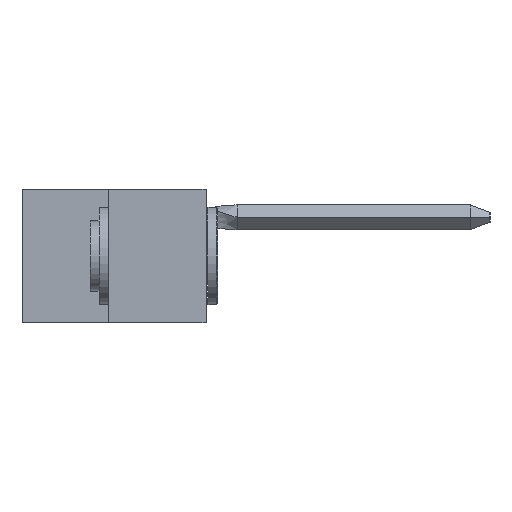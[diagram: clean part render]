
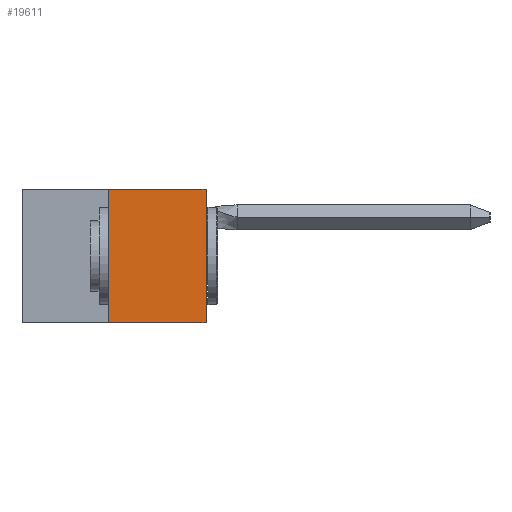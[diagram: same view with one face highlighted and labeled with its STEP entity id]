
A CAD part, left-side view. The second image highlights one B-rep face of the part: STEP entity #19611.
In plain terms, the highlighted planar face has unit normal (-1, 0, 0).
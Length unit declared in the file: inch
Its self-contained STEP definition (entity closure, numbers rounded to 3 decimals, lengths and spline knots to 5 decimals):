
#508 = CARTESIAN_POINT ( 'NONE',  ( 0., 0.473, 0. ) ) ;
#851 = LINE ( 'NONE', #508, #9028 ) ;
#1342 = CARTESIAN_POINT ( 'NONE',  ( 0., 0., 0. ) ) ;
#2151 = LINE ( 'NONE', #45233, #27827 ) ;
#2389 = VECTOR ( 'NONE', #42499, 39.37008 ) ;
#2780 = CARTESIAN_POINT ( 'NONE',  ( 0., 0.25, 0. ) ) ;
#4351 = ORIENTED_EDGE ( 'NONE', *, *, #38464, .F. ) ;
#4510 = EDGE_CURVE ( 'NONE', #21050, #21208, #851, .T. ) ;
#5369 = LINE ( 'NONE', #35914, #32183 ) ;
#5709 = EDGE_CURVE ( 'NONE', #13267, #24226, #6736, .T. ) ;
#6736 = LINE ( 'NONE', #28486, #2389 ) ;
#8425 = EDGE_LOOP ( 'NONE', ( #32876, #4351, #35354, #34177 ) ) ;
#9028 = VECTOR ( 'NONE', #31850, 39.37008 ) ;
#9356 = DIRECTION ( 'NONE',  ( 0., 0., -1. ) ) ;
#9668 = PLANE ( 'NONE',  #33162 ) ;
#11860 = CARTESIAN_POINT ( 'NONE',  ( 0., 0.25, -0.343 ) ) ;
#13267 = VERTEX_POINT ( 'NONE', #11860 ) ;
#19611 = ADVANCED_FACE ( 'NONE', ( #37622 ), #9668, .F. ) ;
#21050 = VERTEX_POINT ( 'NONE', #2780 ) ;
#21208 = VERTEX_POINT ( 'NONE', #1342 ) ;
#23194 = CARTESIAN_POINT ( 'NONE',  ( 0., 0.473, 0. ) ) ;
#24226 = VERTEX_POINT ( 'NONE', #32682 ) ;
#27122 = EDGE_CURVE ( 'NONE', #24226, #21208, #5369, .T. ) ;
#27405 = DIRECTION ( 'NONE',  ( 0., 0., 1. ) ) ;
#27827 = VECTOR ( 'NONE', #27405, 39.37008 ) ;
#28486 = CARTESIAN_POINT ( 'NONE',  ( 0., 0.473, -0.343 ) ) ;
#31850 = DIRECTION ( 'NONE',  ( 0., -1., 0. ) ) ;
#32183 = VECTOR ( 'NONE', #32277, 39.37008 ) ;
#32277 = DIRECTION ( 'NONE',  ( 0., 0., 1. ) ) ;
#32682 = CARTESIAN_POINT ( 'NONE',  ( 0., 0., -0.343 ) ) ;
#32876 = ORIENTED_EDGE ( 'NONE', *, *, #4510, .F. ) ;
#33162 = AXIS2_PLACEMENT_3D ( 'NONE', #23194, #40982, #9356 ) ;
#34177 = ORIENTED_EDGE ( 'NONE', *, *, #27122, .T. ) ;
#35354 = ORIENTED_EDGE ( 'NONE', *, *, #5709, .T. ) ;
#35914 = CARTESIAN_POINT ( 'NONE',  ( 0., 0., 0. ) ) ;
#37622 = FACE_OUTER_BOUND ( 'NONE', #8425, .T. ) ;
#38464 = EDGE_CURVE ( 'NONE', #13267, #21050, #2151, .T. ) ;
#40982 = DIRECTION ( 'NONE',  ( 1., 0., 0. ) ) ;
#42499 = DIRECTION ( 'NONE',  ( 0., -1., 0. ) ) ;
#45233 = CARTESIAN_POINT ( 'NONE',  ( 0., 0.25, 0. ) ) ;
